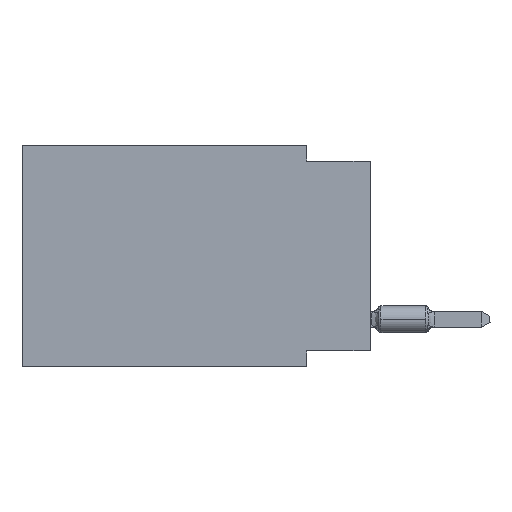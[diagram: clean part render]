
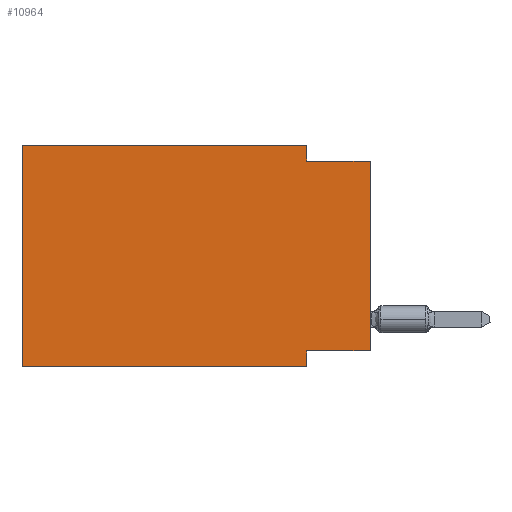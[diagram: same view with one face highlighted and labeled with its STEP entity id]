
A CAD part, left-side view. The second image highlights one B-rep face of the part: STEP entity #10964.
In plain terms, the highlighted planar face has unit normal (-1, 0, 0).
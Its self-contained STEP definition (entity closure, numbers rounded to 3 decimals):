
#627 = EDGE_CURVE ( 'NONE', #43424, #36922, #43131, .T. ) ;
#2705 = LINE ( 'NONE', #45868, #36108 ) ;
#4512 = DIRECTION ( 'NONE',  ( 0., -1., 0. ) ) ;
#4646 = LINE ( 'NONE', #18995, #28053 ) ;
#5298 = ORIENTED_EDGE ( 'NONE', *, *, #9367, .F. ) ;
#6360 = CARTESIAN_POINT ( 'NONE',  ( 0., 2.54, -8.255 ) ) ;
#7022 = CARTESIAN_POINT ( 'NONE',  ( 0., 0., -8.255 ) ) ;
#7431 = ORIENTED_EDGE ( 'NONE', *, *, #35037, .F. ) ;
#7881 = DIRECTION ( 'NONE',  ( 0., 0., 1. ) ) ;
#8107 = ORIENTED_EDGE ( 'NONE', *, *, #627, .F. ) ;
#9176 = VECTOR ( 'NONE', #27537, 1000. ) ;
#9367 = EDGE_CURVE ( 'NONE', #22399, #17861, #16311, .T. ) ;
#10964 = ADVANCED_FACE ( 'NONE', ( #22993 ), #41340, .F. ) ;
#12089 = DIRECTION ( 'NONE',  ( 0., 0., -1. ) ) ;
#12199 = VERTEX_POINT ( 'NONE', #45073 ) ;
#13373 = CARTESIAN_POINT ( 'NONE',  ( 0., 13.97, 0. ) ) ;
#16181 = VECTOR ( 'NONE', #4512, 1000. ) ;
#16311 = LINE ( 'NONE', #18868, #21710 ) ;
#17861 = VERTEX_POINT ( 'NONE', #36089 ) ;
#18241 = LINE ( 'NONE', #22209, #38071 ) ;
#18245 = DIRECTION ( 'NONE',  ( 0., 0., -1. ) ) ;
#18868 = CARTESIAN_POINT ( 'NONE',  ( 0., 13.97, 0. ) ) ;
#18995 = CARTESIAN_POINT ( 'NONE',  ( 0., 0., 0. ) ) ;
#19552 = DIRECTION ( 'NONE',  ( 0., -1., 0. ) ) ;
#19717 = CARTESIAN_POINT ( 'NONE',  ( 0., 13.97, 0. ) ) ;
#20295 = EDGE_CURVE ( 'NONE', #12199, #22399, #45204, .T. ) ;
#21374 = EDGE_CURVE ( 'NONE', #45813, #36112, #18241, .T. ) ;
#21506 = ORIENTED_EDGE ( 'NONE', *, *, #27843, .F. ) ;
#21710 = VECTOR ( 'NONE', #19552, 1000. ) ;
#22134 = LINE ( 'NONE', #36304, #16181 ) ;
#22209 = CARTESIAN_POINT ( 'NONE',  ( 0., 0., -0.635 ) ) ;
#22399 = VERTEX_POINT ( 'NONE', #41833 ) ;
#22993 = FACE_OUTER_BOUND ( 'NONE', #38382, .T. ) ;
#23018 = VECTOR ( 'NONE', #27875, 1000. ) ;
#27259 = EDGE_CURVE ( 'NONE', #12199, #36922, #22134, .T. ) ;
#27537 = DIRECTION ( 'NONE',  ( 0., 0., 1. ) ) ;
#27843 = EDGE_CURVE ( 'NONE', #34431, #43424, #35073, .T. ) ;
#27875 = DIRECTION ( 'NONE',  ( 0., 1., 0. ) ) ;
#28053 = VECTOR ( 'NONE', #7881, 1000. ) ;
#29669 = CARTESIAN_POINT ( 'NONE',  ( 0., 2.54, -8.89 ) ) ;
#29947 = CARTESIAN_POINT ( 'NONE',  ( 0., 0., -0.635 ) ) ;
#30148 = ORIENTED_EDGE ( 'NONE', *, *, #20295, .F. ) ;
#30266 = VECTOR ( 'NONE', #18245, 1000. ) ;
#30434 = DIRECTION ( 'NONE',  ( 1., 0., 0. ) ) ;
#30627 = ORIENTED_EDGE ( 'NONE', *, *, #21374, .F. ) ;
#31241 = DIRECTION ( 'NONE',  ( 0., 0., -1. ) ) ;
#34431 = VERTEX_POINT ( 'NONE', #7022 ) ;
#35037 = EDGE_CURVE ( 'NONE', #17861, #45813, #2705, .T. ) ;
#35073 = LINE ( 'NONE', #38572, #23018 ) ;
#35433 = CARTESIAN_POINT ( 'NONE',  ( 0., 2.54, -8.89 ) ) ;
#35476 = ORIENTED_EDGE ( 'NONE', *, *, #27259, .T. ) ;
#36035 = EDGE_CURVE ( 'NONE', #34431, #36112, #4646, .T. ) ;
#36089 = CARTESIAN_POINT ( 'NONE',  ( 0., 2.54, 0. ) ) ;
#36108 = VECTOR ( 'NONE', #31241, 1000. ) ;
#36112 = VERTEX_POINT ( 'NONE', #29947 ) ;
#36210 = ORIENTED_EDGE ( 'NONE', *, *, #36035, .T. ) ;
#36304 = CARTESIAN_POINT ( 'NONE',  ( 0., 13.97, -8.89 ) ) ;
#36382 = DIRECTION ( 'NONE',  ( 0., -1., 0. ) ) ;
#36922 = VERTEX_POINT ( 'NONE', #35433 ) ;
#37330 = AXIS2_PLACEMENT_3D ( 'NONE', #19717, #30434, #12089 ) ;
#38071 = VECTOR ( 'NONE', #36382, 1000. ) ;
#38382 = EDGE_LOOP ( 'NONE', ( #36210, #30627, #7431, #5298, #30148, #35476, #8107, #21506 ) ) ;
#38572 = CARTESIAN_POINT ( 'NONE',  ( 0., 0., -8.255 ) ) ;
#41340 = PLANE ( 'NONE',  #37330 ) ;
#41493 = CARTESIAN_POINT ( 'NONE',  ( 0., 2.54, -0.635 ) ) ;
#41833 = CARTESIAN_POINT ( 'NONE',  ( 0., 13.97, 0. ) ) ;
#43131 = LINE ( 'NONE', #29669, #30266 ) ;
#43424 = VERTEX_POINT ( 'NONE', #6360 ) ;
#45073 = CARTESIAN_POINT ( 'NONE',  ( 0., 13.97, -8.89 ) ) ;
#45204 = LINE ( 'NONE', #13373, #9176 ) ;
#45813 = VERTEX_POINT ( 'NONE', #41493 ) ;
#45868 = CARTESIAN_POINT ( 'NONE',  ( 0., 2.54, 0. ) ) ;
